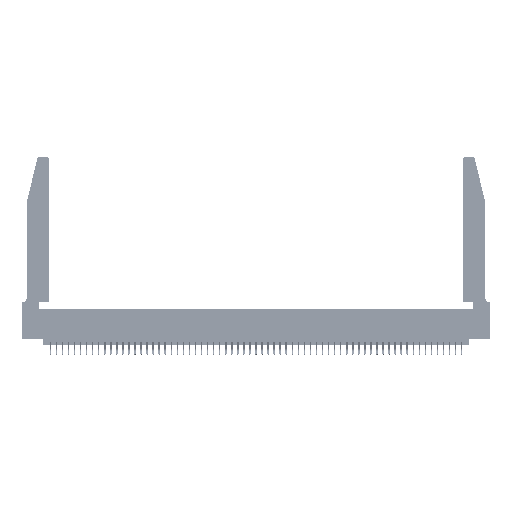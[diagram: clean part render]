
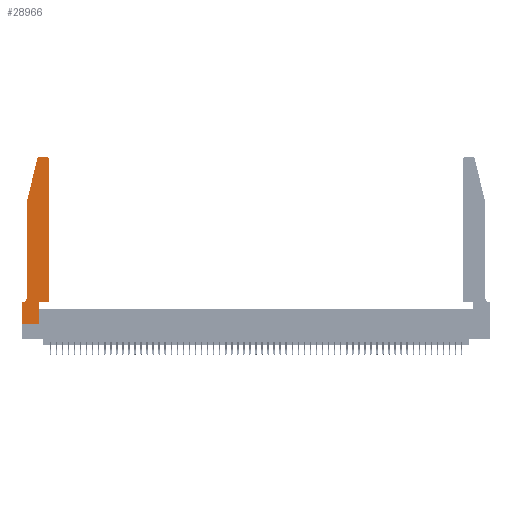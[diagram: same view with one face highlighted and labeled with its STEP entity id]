
A CAD part, top view. The second image highlights one B-rep face of the part: STEP entity #28966.
In plain terms, the highlighted planar face has unit normal (0, 0, 1).
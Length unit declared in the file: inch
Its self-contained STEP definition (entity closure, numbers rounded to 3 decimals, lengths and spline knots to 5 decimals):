
#161 = CARTESIAN_POINT ( 'NONE',  ( 0., 0.35, 0.37 ) ) ;
#682 = ORIENTED_EDGE ( 'NONE', *, *, #13629, .T. ) ;
#844 = CARTESIAN_POINT ( 'NONE',  ( 0.0755, 2., 0.37 ) ) ;
#2807 = VECTOR ( 'NONE', #5159, 39.37008 ) ;
#2882 = VERTEX_POINT ( 'NONE', #24859 ) ;
#3253 = CARTESIAN_POINT ( 'NONE',  ( 0.4505, 0.35, 0.37 ) ) ;
#5138 = DIRECTION ( 'NONE',  ( 1., 0., 0. ) ) ;
#5159 = DIRECTION ( 'NONE',  ( 0., -1., 0. ) ) ;
#5379 = ORIENTED_EDGE ( 'NONE', *, *, #22504, .T. ) ;
#5615 = EDGE_CURVE ( 'NONE', #10012, #51238, #49000, .T. ) ;
#6621 = DIRECTION ( 'NONE',  ( 0., 0., 1. ) ) ;
#6736 = CARTESIAN_POINT ( 'NONE',  ( 0.0755, 0.42, 0.37 ) ) ;
#7152 = DIRECTION ( 'NONE',  ( 0., 0., -1. ) ) ;
#7289 = CARTESIAN_POINT ( 'NONE',  ( 0., 0., 0.37 ) ) ;
#7319 = VERTEX_POINT ( 'NONE', #8667 ) ;
#7873 = ORIENTED_EDGE ( 'NONE', *, *, #32858, .T. ) ;
#8607 = VERTEX_POINT ( 'NONE', #37874 ) ;
#8667 = CARTESIAN_POINT ( 'NONE',  ( 0.4505, 2.72, 0.37 ) ) ;
#9460 = EDGE_CURVE ( 'NONE', #8607, #2882, #21120, .T. ) ;
#9598 = CARTESIAN_POINT ( 'NONE',  ( 0.284, 2.75, 0.37 ) ) ;
#10012 = VERTEX_POINT ( 'NONE', #21945 ) ;
#10427 = AXIS2_PLACEMENT_3D ( 'NONE', #32399, #6621, #36700 ) ;
#10835 = CARTESIAN_POINT ( 'NONE',  ( 0., 0.35, 0.37 ) ) ;
#11060 = CARTESIAN_POINT ( 'NONE',  ( 0.0055, 0.35, 0.37 ) ) ;
#11565 = VECTOR ( 'NONE', #37673, 39.37008 ) ;
#11869 = VECTOR ( 'NONE', #37374, 39.37008 ) ;
#12331 = CARTESIAN_POINT ( 'NONE',  ( 0., 0., 0.37 ) ) ;
#12658 = VECTOR ( 'NONE', #30594, 39.37008 ) ;
#12787 = AXIS2_PLACEMENT_3D ( 'NONE', #25752, #7152, #30073 ) ;
#12971 = ORIENTED_EDGE ( 'NONE', *, *, #33275, .T. ) ;
#13104 = AXIS2_PLACEMENT_3D ( 'NONE', #10835, #23776, #53829 ) ;
#13466 = VERTEX_POINT ( 'NONE', #11060 ) ;
#13629 = EDGE_CURVE ( 'NONE', #7319, #13663, #42926, .T. ) ;
#13663 = VERTEX_POINT ( 'NONE', #37705 ) ;
#14059 = ORIENTED_EDGE ( 'NONE', *, *, #29893, .T. ) ;
#14259 = ORIENTED_EDGE ( 'NONE', *, *, #32127, .T. ) ;
#15727 = CARTESIAN_POINT ( 'NONE',  ( 0.0755, 2., 0.37 ) ) ;
#16465 = DIRECTION ( 'NONE',  ( 1., 0., 0. ) ) ;
#16661 = FACE_OUTER_BOUND ( 'NONE', #40656, .T. ) ;
#20111 = ORIENTED_EDGE ( 'NONE', *, *, #5615, .T. ) ;
#21120 = LINE ( 'NONE', #30305, #27189 ) ;
#21556 = CIRCLE ( 'NONE', #10427, 0.03 ) ;
#21945 = CARTESIAN_POINT ( 'NONE',  ( 0.25487, 2.72718, 0.37 ) ) ;
#22504 = EDGE_CURVE ( 'NONE', #13663, #34821, #45845, .T. ) ;
#23017 = EDGE_CURVE ( 'NONE', #34821, #10012, #21556, .T. ) ;
#23289 = LINE ( 'NONE', #7289, #11869 ) ;
#23776 = DIRECTION ( 'NONE',  ( 0., 0., 1. ) ) ;
#24327 = LINE ( 'NONE', #844, #2807 ) ;
#24746 = EDGE_CURVE ( 'NONE', #41284, #8607, #29202, .T. ) ;
#24859 = CARTESIAN_POINT ( 'NONE',  ( 0.2865, 0.35, 0.37 ) ) ;
#24910 = CARTESIAN_POINT ( 'NONE',  ( 0.4205, 2.72, 0.37 ) ) ;
#25729 = ORIENTED_EDGE ( 'NONE', *, *, #49187, .T. ) ;
#25752 = CARTESIAN_POINT ( 'NONE',  ( 0.0055, 0.42, 0.37 ) ) ;
#26257 = CARTESIAN_POINT ( 'NONE',  ( 0.4505, 0.35, 0.37 ) ) ;
#27189 = VECTOR ( 'NONE', #34644, 39.37008 ) ;
#27405 = EDGE_CURVE ( 'NONE', #13466, #45741, #35618, .T. ) ;
#28461 = VERTEX_POINT ( 'NONE', #6736 ) ;
#28966 = ADVANCED_FACE ( 'NONE', ( #16661 ), #49492, .T. ) ;
#29202 = LINE ( 'NONE', #12331, #39251 ) ;
#29228 = CARTESIAN_POINT ( 'NONE',  ( 0.0755, 0.35, 0.37 ) ) ;
#29269 = DIRECTION ( 'NONE',  ( 1., 0., 0. ) ) ;
#29893 = EDGE_CURVE ( 'NONE', #28461, #13466, #32081, .T. ) ;
#30073 = DIRECTION ( 'NONE',  ( -1., 0., 0. ) ) ;
#30305 = CARTESIAN_POINT ( 'NONE',  ( 0.2865, 0.35, 0.37 ) ) ;
#30594 = DIRECTION ( 'NONE',  ( 0., 1., 0. ) ) ;
#32081 = CIRCLE ( 'NONE', #12787, 0.07 ) ;
#32127 = EDGE_CURVE ( 'NONE', #36586, #7319, #45603, .T. ) ;
#32399 = CARTESIAN_POINT ( 'NONE',  ( 0.284, 2.72, 0.37 ) ) ;
#32858 = EDGE_CURVE ( 'NONE', #2882, #36586, #33457, .T. ) ;
#33275 = EDGE_CURVE ( 'NONE', #45741, #41284, #23289, .T. ) ;
#33457 = LINE ( 'NONE', #35239, #54942 ) ;
#34644 = DIRECTION ( 'NONE',  ( 0., 1., 0. ) ) ;
#34821 = VERTEX_POINT ( 'NONE', #9598 ) ;
#35239 = CARTESIAN_POINT ( 'NONE',  ( 0.4505, 0.35, 0.37 ) ) ;
#35618 = LINE ( 'NONE', #29228, #45661 ) ;
#36586 = VERTEX_POINT ( 'NONE', #3253 ) ;
#36700 = DIRECTION ( 'NONE',  ( 1., 0., 0. ) ) ;
#37374 = DIRECTION ( 'NONE',  ( 0., -1., 0. ) ) ;
#37673 = DIRECTION ( 'NONE',  ( -1., 0., 0. ) ) ;
#37705 = CARTESIAN_POINT ( 'NONE',  ( 0.4205, 2.75, 0.37 ) ) ;
#37874 = CARTESIAN_POINT ( 'NONE',  ( 0.2865, 0., 0.37 ) ) ;
#38927 = VECTOR ( 'NONE', #45783, 39.37008 ) ;
#39251 = VECTOR ( 'NONE', #16465, 39.37008 ) ;
#39767 = ORIENTED_EDGE ( 'NONE', *, *, #24746, .T. ) ;
#40656 = EDGE_LOOP ( 'NONE', ( #5379, #41040, #20111, #25729, #14059, #46556, #12971, #39767, #52245, #7873, #14259, #682 ) ) ;
#41040 = ORIENTED_EDGE ( 'NONE', *, *, #23017, .T. ) ;
#41284 = VERTEX_POINT ( 'NONE', #49064 ) ;
#41996 = CARTESIAN_POINT ( 'NONE',  ( 0.2605, 2.75, 0.37 ) ) ;
#42500 = AXIS2_PLACEMENT_3D ( 'NONE', #24910, #54959, #29269 ) ;
#42926 = CIRCLE ( 'NONE', #42500, 0.03 ) ;
#45603 = LINE ( 'NONE', #26257, #12658 ) ;
#45661 = VECTOR ( 'NONE', #46457, 39.37008 ) ;
#45741 = VERTEX_POINT ( 'NONE', #161 ) ;
#45783 = DIRECTION ( 'NONE',  ( -0.239, -0.971, 0. ) ) ;
#45845 = LINE ( 'NONE', #41996, #11565 ) ;
#46457 = DIRECTION ( 'NONE',  ( -1., 0., 0. ) ) ;
#46556 = ORIENTED_EDGE ( 'NONE', *, *, #27405, .T. ) ;
#49000 = LINE ( 'NONE', #15727, #38927 ) ;
#49064 = CARTESIAN_POINT ( 'NONE',  ( 0., 0., 0.37 ) ) ;
#49187 = EDGE_CURVE ( 'NONE', #51238, #28461, #24327, .T. ) ;
#49492 = PLANE ( 'NONE',  #13104 ) ;
#51238 = VERTEX_POINT ( 'NONE', #54832 ) ;
#52245 = ORIENTED_EDGE ( 'NONE', *, *, #9460, .T. ) ;
#53829 = DIRECTION ( 'NONE',  ( 1., 0., 0. ) ) ;
#54832 = CARTESIAN_POINT ( 'NONE',  ( 0.0755, 2., 0.37 ) ) ;
#54942 = VECTOR ( 'NONE', #5138, 39.37008 ) ;
#54959 = DIRECTION ( 'NONE',  ( 0., 0., 1. ) ) ;
